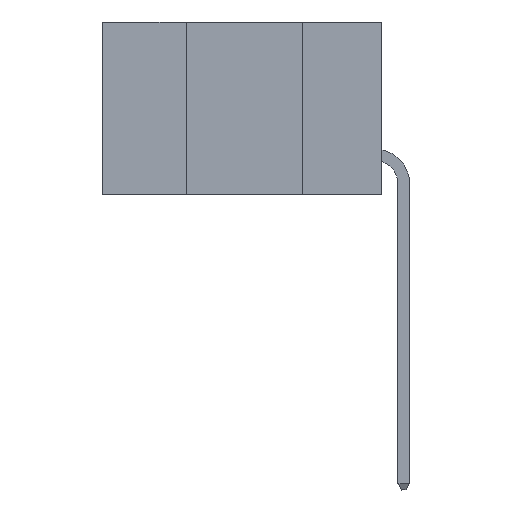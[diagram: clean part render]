
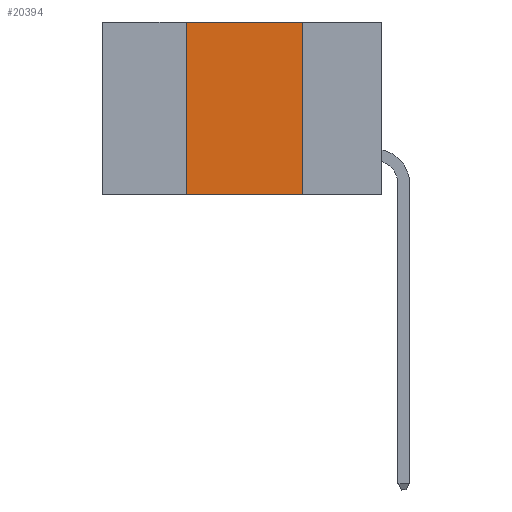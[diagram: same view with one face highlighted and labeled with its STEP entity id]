
A CAD part, left-side view. The second image highlights one B-rep face of the part: STEP entity #20394.
In plain terms, the highlighted planar face has unit normal (-1, 0, 0).
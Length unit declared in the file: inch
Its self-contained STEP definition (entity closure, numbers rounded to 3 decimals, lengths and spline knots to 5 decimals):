
#543 = EDGE_CURVE ( 'NONE', #19880, #36120, #5207, .T. ) ;
#1286 = VERTEX_POINT ( 'NONE', #7786 ) ;
#2321 = VECTOR ( 'NONE', #25232, 39.37008 ) ;
#3376 = EDGE_CURVE ( 'NONE', #36120, #1286, #37622, .T. ) ;
#4429 = CARTESIAN_POINT ( 'NONE',  ( 0., 0.6, -0.37 ) ) ;
#5200 = VERTEX_POINT ( 'NONE', #17155 ) ;
#5207 = LINE ( 'NONE', #16418, #2321 ) ;
#7128 = CARTESIAN_POINT ( 'NONE',  ( 0., 0.17, 0. ) ) ;
#7156 = ORIENTED_EDGE ( 'NONE', *, *, #14368, .F. ) ;
#7786 = CARTESIAN_POINT ( 'NONE',  ( 0., 0.17, -0.37 ) ) ;
#9127 = EDGE_LOOP ( 'NONE', ( #37103, #20989, #7156, #37387 ) ) ;
#9184 = VECTOR ( 'NONE', #16076, 39.37008 ) ;
#14200 = AXIS2_PLACEMENT_3D ( 'NONE', #31813, #20024, #19499 ) ;
#14368 = EDGE_CURVE ( 'NONE', #5200, #19880, #24109, .T. ) ;
#16076 = DIRECTION ( 'NONE',  ( 0., -1., 0. ) ) ;
#16418 = CARTESIAN_POINT ( 'NONE',  ( 0., 0.6, 0. ) ) ;
#17155 = CARTESIAN_POINT ( 'NONE',  ( 0., 0.42, -0.37 ) ) ;
#19499 = DIRECTION ( 'NONE',  ( 0., 0., -1. ) ) ;
#19880 = VERTEX_POINT ( 'NONE', #29600 ) ;
#20024 = DIRECTION ( 'NONE',  ( 1., 0., 0. ) ) ;
#20394 = ADVANCED_FACE ( 'NONE', ( #35240 ), #38117, .F. ) ;
#20989 = ORIENTED_EDGE ( 'NONE', *, *, #543, .F. ) ;
#23947 = VECTOR ( 'NONE', #28611, 39.37008 ) ;
#24109 = LINE ( 'NONE', #28135, #27911 ) ;
#24469 = CARTESIAN_POINT ( 'NONE',  ( 0., 0.17, 0. ) ) ;
#25232 = DIRECTION ( 'NONE',  ( 0., -1., 0. ) ) ;
#25352 = DIRECTION ( 'NONE',  ( 0., 0., 1. ) ) ;
#27911 = VECTOR ( 'NONE', #25352, 39.37008 ) ;
#28135 = CARTESIAN_POINT ( 'NONE',  ( 0., 0.42, 0. ) ) ;
#28611 = DIRECTION ( 'NONE',  ( 0., 0., -1. ) ) ;
#29600 = CARTESIAN_POINT ( 'NONE',  ( 0., 0.42, 0. ) ) ;
#31813 = CARTESIAN_POINT ( 'NONE',  ( 0., 0.6, 0. ) ) ;
#35240 = FACE_OUTER_BOUND ( 'NONE', #9127, .T. ) ;
#35736 = EDGE_CURVE ( 'NONE', #5200, #1286, #37110, .T. ) ;
#36120 = VERTEX_POINT ( 'NONE', #24469 ) ;
#37103 = ORIENTED_EDGE ( 'NONE', *, *, #3376, .F. ) ;
#37110 = LINE ( 'NONE', #4429, #9184 ) ;
#37387 = ORIENTED_EDGE ( 'NONE', *, *, #35736, .T. ) ;
#37622 = LINE ( 'NONE', #7128, #23947 ) ;
#38117 = PLANE ( 'NONE',  #14200 ) ;
